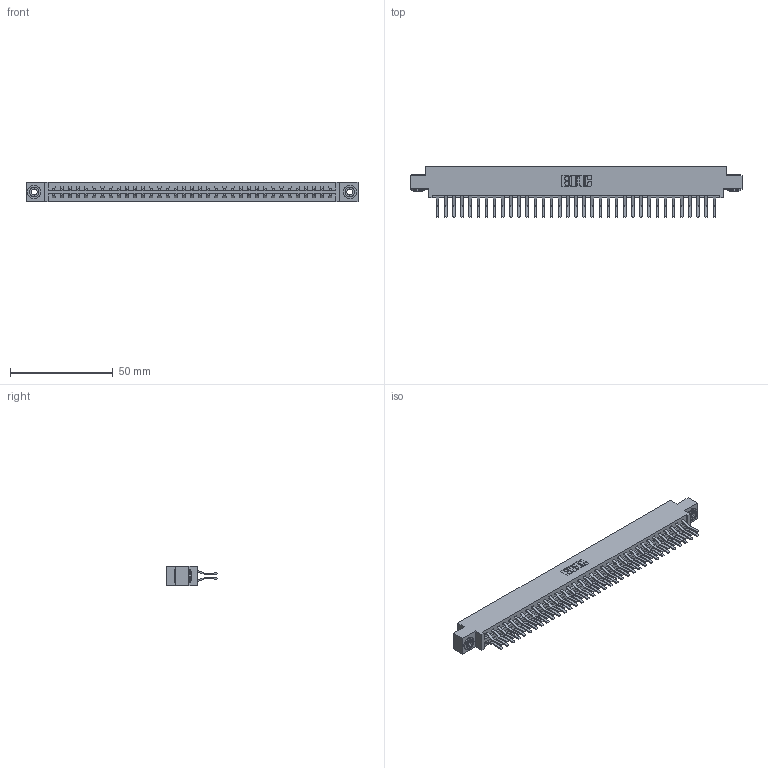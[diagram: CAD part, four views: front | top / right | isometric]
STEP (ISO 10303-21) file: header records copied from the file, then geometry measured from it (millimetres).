
FILE_DESCRIPTION (( 'STEP AP203' ), '1' );
FILE_NAME ('337-070-560-803.STEP', '2019-10-15T11:19:40', ( '' ), ( '' ), 'SwSTEP 2.0', 'SolidWorks 2016', '' );
FILE_SCHEMA (( 'CONFIG_CONTROL_DESIGN' ));
Length unit declared in the file: inch
Products named in the file (4): 337-070-560-803; 345-250-002_345-250-002-102; 337 Part_0.170 Offset - 0.156 Dia-TH; 345-292-001_560 Tail
Assembly tree (73 placements, depth 2):
  337-070-560-803
    337 Part_0.170 Offset - 0.156 Dia-TH
    345-292-001_560 Tail  x70
    345-250-002_345-250-002-102  x2
Bounding box: 161.7 x 24.78 x 9.4 mm (x, y, z)
Volume: 17308.4 mm3; surface area: 21159.3 mm2
Topology: 73 solids, 73 shells, 4076 faces, 12089 edges, 7962 vertices
Faces by surface type: plane 2744, cylinder 1324, cone 8
Entity records: 28912 total; most frequent: CARTESIAN_POINT 4853, ORIENTED_EDGE 4782, DIRECTION 4177, EDGE_CURVE 2391, LINE 2235, VECTOR 2235, VERTEX_POINT 1590, AXIS2_PLACEMENT_3D 971
